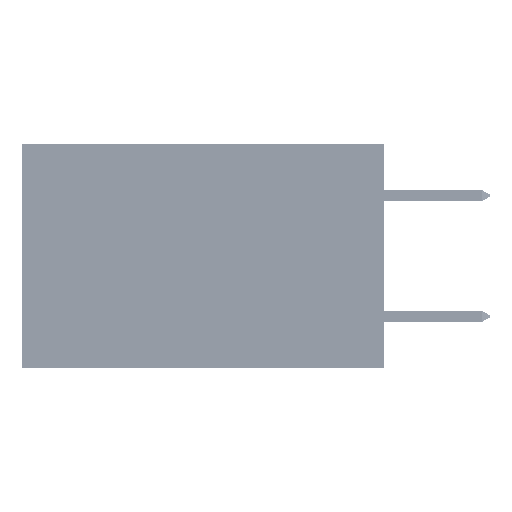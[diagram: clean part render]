
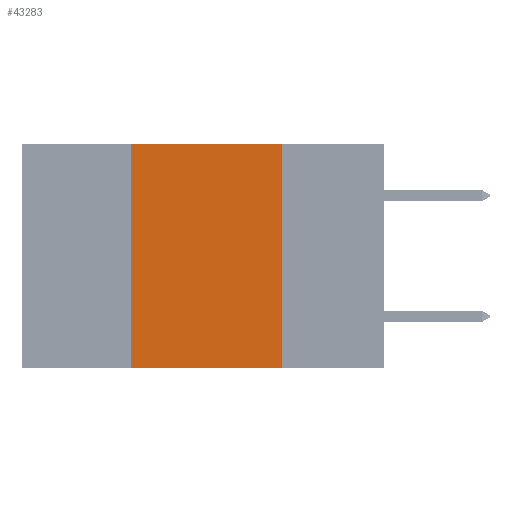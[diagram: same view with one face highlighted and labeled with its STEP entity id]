
A CAD part, left-side view. The second image highlights one B-rep face of the part: STEP entity #43283.
In plain terms, the highlighted planar face has unit normal (-1, 0, 0).
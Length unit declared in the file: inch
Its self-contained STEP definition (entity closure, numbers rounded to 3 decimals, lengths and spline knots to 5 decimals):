
#2792 = LINE ( 'NONE', #7471, #34547 ) ;
#2882 = ORIENTED_EDGE ( 'NONE', *, *, #45042, .T. ) ;
#4223 = EDGE_CURVE ( 'NONE', #37979, #7513, #7697, .T. ) ;
#6441 = VECTOR ( 'NONE', #18686, 39.37008 ) ;
#7323 = VECTOR ( 'NONE', #8580, 39.37008 ) ;
#7402 = CARTESIAN_POINT ( 'NONE',  ( 0., 0.42, 0. ) ) ;
#7471 = CARTESIAN_POINT ( 'NONE',  ( 0., 0.6, -0.37 ) ) ;
#7513 = VERTEX_POINT ( 'NONE', #7402 ) ;
#7697 = LINE ( 'NONE', #10666, #33017 ) ;
#8580 = DIRECTION ( 'NONE',  ( 0., -1., 0. ) ) ;
#10508 = FACE_OUTER_BOUND ( 'NONE', #42612, .T. ) ;
#10567 = CARTESIAN_POINT ( 'NONE',  ( 0., 0.17, -0.37 ) ) ;
#10666 = CARTESIAN_POINT ( 'NONE',  ( 0., 0.42, 0. ) ) ;
#14561 = DIRECTION ( 'NONE',  ( 0., -1., 0. ) ) ;
#14718 = DIRECTION ( 'NONE',  ( 1., 0., 0. ) ) ;
#15054 = EDGE_CURVE ( 'NONE', #32355, #15559, #32875, .T. ) ;
#15559 = VERTEX_POINT ( 'NONE', #10567 ) ;
#18686 = DIRECTION ( 'NONE',  ( 0., 0., -1. ) ) ;
#19494 = CARTESIAN_POINT ( 'NONE',  ( 0., 0.6, 0. ) ) ;
#19831 = CARTESIAN_POINT ( 'NONE',  ( 0., 0.42, -0.37 ) ) ;
#20596 = EDGE_CURVE ( 'NONE', #7513, #32355, #47982, .T. ) ;
#22193 = DIRECTION ( 'NONE',  ( 0., 0., 1. ) ) ;
#22324 = ORIENTED_EDGE ( 'NONE', *, *, #15054, .F. ) ;
#26559 = PLANE ( 'NONE',  #39895 ) ;
#30515 = CARTESIAN_POINT ( 'NONE',  ( 0., 0.6, 0. ) ) ;
#32355 = VERTEX_POINT ( 'NONE', #34309 ) ;
#32875 = LINE ( 'NONE', #48599, #6441 ) ;
#33017 = VECTOR ( 'NONE', #22193, 39.37008 ) ;
#34309 = CARTESIAN_POINT ( 'NONE',  ( 0., 0.17, 0. ) ) ;
#34547 = VECTOR ( 'NONE', #14561, 39.37008 ) ;
#36245 = ORIENTED_EDGE ( 'NONE', *, *, #20596, .F. ) ;
#37979 = VERTEX_POINT ( 'NONE', #19831 ) ;
#39895 = AXIS2_PLACEMENT_3D ( 'NONE', #30515, #14718, #41021 ) ;
#41021 = DIRECTION ( 'NONE',  ( 0., 0., -1. ) ) ;
#42612 = EDGE_LOOP ( 'NONE', ( #22324, #36245, #46996, #2882 ) ) ;
#43283 = ADVANCED_FACE ( 'NONE', ( #10508 ), #26559, .F. ) ;
#45042 = EDGE_CURVE ( 'NONE', #37979, #15559, #2792, .T. ) ;
#46996 = ORIENTED_EDGE ( 'NONE', *, *, #4223, .F. ) ;
#47982 = LINE ( 'NONE', #19494, #7323 ) ;
#48599 = CARTESIAN_POINT ( 'NONE',  ( 0., 0.17, 0. ) ) ;
